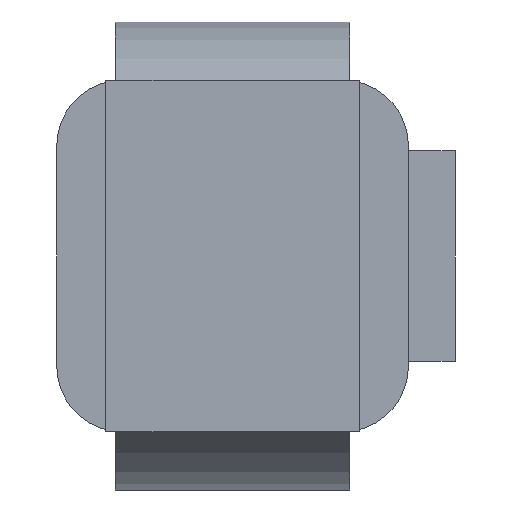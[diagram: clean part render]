
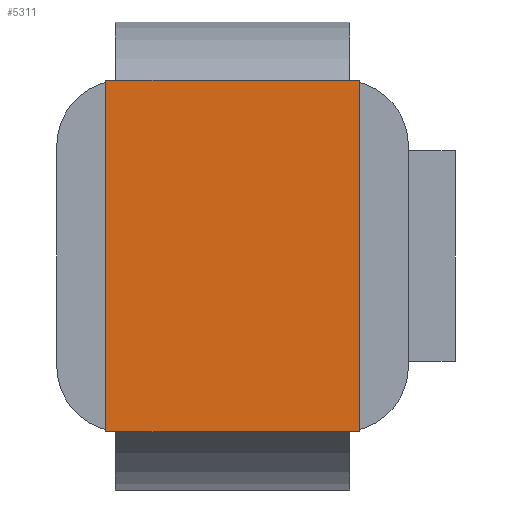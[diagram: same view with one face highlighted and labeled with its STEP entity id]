
A CAD part, front view. The second image highlights one B-rep face of the part: STEP entity #5311.
In plain terms, the highlighted planar face has unit normal (0, -1, 0).
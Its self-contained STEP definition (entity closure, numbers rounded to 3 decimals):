
#1319 = PLANE('',#1320);
#1320 = AXIS2_PLACEMENT_3D('',#1321,#1322,#1323);
#1321 = CARTESIAN_POINT('',(0.,2.6,15.));
#1322 = DIRECTION('',(0.,0.,-1.));
#1323 = DIRECTION('',(-1.,0.,0.));
#1437 = PLANE('',#1438);
#1438 = AXIS2_PLACEMENT_3D('',#1439,#1440,#1441);
#1439 = CARTESIAN_POINT('',(0.,2.6,0.));
#1440 = DIRECTION('',(0.,0.,-1.));
#1441 = DIRECTION('',(-1.,0.,0.));
#2606 = VERTEX_POINT('',#2607);
#2607 = CARTESIAN_POINT('',(3.5,-5.8,0.));
#2621 = PLANE('',#2622);
#2622 = AXIS2_PLACEMENT_3D('',#2623,#2624,#2625);
#2623 = CARTESIAN_POINT('',(3.5,0.,0.));
#2624 = DIRECTION('',(1.,0.,0.));
#2625 = DIRECTION('',(0.,-1.,0.));
#2633 = EDGE_CURVE('',#2606,#2634,#2636,.T.);
#2634 = VERTEX_POINT('',#2635);
#2635 = CARTESIAN_POINT('',(-7.3,-5.8,0.));
#2636 = SURFACE_CURVE('',#2637,(#2641,#2648),.PCURVE_S1.);
#2637 = LINE('',#2638,#2639);
#2638 = CARTESIAN_POINT('',(3.5,-5.8,0.));
#2639 = VECTOR('',#2640,1.);
#2640 = DIRECTION('',(-1.,0.,0.));
#2641 = PCURVE('',#1437,#2642);
#2642 = DEFINITIONAL_REPRESENTATION('',(#2643),#2647);
#2643 = LINE('',#2644,#2645);
#2644 = CARTESIAN_POINT('',(-3.5,-8.4));
#2645 = VECTOR('',#2646,1.);
#2646 = DIRECTION('',(1.,0.));
#2647 = ( GEOMETRIC_REPRESENTATION_CONTEXT(2) 
PARAMETRIC_REPRESENTATION_CONTEXT() REPRESENTATION_CONTEXT('2D SPACE',''
  ) );
#2648 = PCURVE('',#2649,#2654);
#2649 = PLANE('',#2650);
#2650 = AXIS2_PLACEMENT_3D('',#2651,#2652,#2653);
#2651 = CARTESIAN_POINT('',(3.5,-5.8,0.));
#2652 = DIRECTION('',(0.,-1.,0.));
#2653 = DIRECTION('',(-1.,0.,0.));
#2654 = DEFINITIONAL_REPRESENTATION('',(#2655),#2659);
#2655 = LINE('',#2656,#2657);
#2656 = CARTESIAN_POINT('',(0.,0.));
#2657 = VECTOR('',#2658,1.);
#2658 = DIRECTION('',(1.,0.));
#2659 = ( GEOMETRIC_REPRESENTATION_CONTEXT(2) 
PARAMETRIC_REPRESENTATION_CONTEXT() REPRESENTATION_CONTEXT('2D SPACE',''
  ) );
#2677 = PLANE('',#2678);
#2678 = AXIS2_PLACEMENT_3D('',#2679,#2680,#2681);
#2679 = CARTESIAN_POINT('',(-7.3,-5.8,0.));
#2680 = DIRECTION('',(-1.,0.,0.));
#2681 = DIRECTION('',(0.,1.,0.));
#2899 = VERTEX_POINT('',#2900);
#2900 = CARTESIAN_POINT('',(3.5,-5.8,15.));
#2921 = EDGE_CURVE('',#2899,#2922,#2924,.T.);
#2922 = VERTEX_POINT('',#2923);
#2923 = CARTESIAN_POINT('',(-7.3,-5.8,15.));
#2924 = SURFACE_CURVE('',#2925,(#2929,#2936),.PCURVE_S1.);
#2925 = LINE('',#2926,#2927);
#2926 = CARTESIAN_POINT('',(3.5,-5.8,15.));
#2927 = VECTOR('',#2928,1.);
#2928 = DIRECTION('',(-1.,0.,0.));
#2929 = PCURVE('',#1319,#2930);
#2930 = DEFINITIONAL_REPRESENTATION('',(#2931),#2935);
#2931 = LINE('',#2932,#2933);
#2932 = CARTESIAN_POINT('',(-3.5,-8.4));
#2933 = VECTOR('',#2934,1.);
#2934 = DIRECTION('',(1.,0.));
#2935 = ( GEOMETRIC_REPRESENTATION_CONTEXT(2) 
PARAMETRIC_REPRESENTATION_CONTEXT() REPRESENTATION_CONTEXT('2D SPACE',''
  ) );
#2936 = PCURVE('',#2649,#2937);
#2937 = DEFINITIONAL_REPRESENTATION('',(#2938),#2942);
#2938 = LINE('',#2939,#2940);
#2939 = CARTESIAN_POINT('',(0.,-15.));
#2940 = VECTOR('',#2941,1.);
#2941 = DIRECTION('',(1.,0.));
#2942 = ( GEOMETRIC_REPRESENTATION_CONTEXT(2) 
PARAMETRIC_REPRESENTATION_CONTEXT() REPRESENTATION_CONTEXT('2D SPACE',''
  ) );
#5288 = EDGE_CURVE('',#2634,#2922,#5289,.T.);
#5289 = SURFACE_CURVE('',#5290,(#5294,#5301),.PCURVE_S1.);
#5290 = LINE('',#5291,#5292);
#5291 = CARTESIAN_POINT('',(-7.3,-5.8,0.));
#5292 = VECTOR('',#5293,1.);
#5293 = DIRECTION('',(0.,0.,1.));
#5294 = PCURVE('',#2677,#5295);
#5295 = DEFINITIONAL_REPRESENTATION('',(#5296),#5300);
#5296 = LINE('',#5297,#5298);
#5297 = CARTESIAN_POINT('',(0.,0.));
#5298 = VECTOR('',#5299,1.);
#5299 = DIRECTION('',(0.,-1.));
#5300 = ( GEOMETRIC_REPRESENTATION_CONTEXT(2) 
PARAMETRIC_REPRESENTATION_CONTEXT() REPRESENTATION_CONTEXT('2D SPACE',''
  ) );
#5301 = PCURVE('',#2649,#5302);
#5302 = DEFINITIONAL_REPRESENTATION('',(#5303),#5307);
#5303 = LINE('',#5304,#5305);
#5304 = CARTESIAN_POINT('',(10.8,0.));
#5305 = VECTOR('',#5306,1.);
#5306 = DIRECTION('',(0.,-1.));
#5307 = ( GEOMETRIC_REPRESENTATION_CONTEXT(2) 
PARAMETRIC_REPRESENTATION_CONTEXT() REPRESENTATION_CONTEXT('2D SPACE',''
  ) );
#5311 = ADVANCED_FACE('',(#5312),#2649,.T.);
#5312 = FACE_BOUND('',#5313,.T.);
#5313 = EDGE_LOOP('',(#5314,#5335,#5336,#5337));
#5314 = ORIENTED_EDGE('',*,*,#5315,.T.);
#5315 = EDGE_CURVE('',#2606,#2899,#5316,.T.);
#5316 = SURFACE_CURVE('',#5317,(#5321,#5328),.PCURVE_S1.);
#5317 = LINE('',#5318,#5319);
#5318 = CARTESIAN_POINT('',(3.5,-5.8,0.));
#5319 = VECTOR('',#5320,1.);
#5320 = DIRECTION('',(0.,0.,1.));
#5321 = PCURVE('',#2649,#5322);
#5322 = DEFINITIONAL_REPRESENTATION('',(#5323),#5327);
#5323 = LINE('',#5324,#5325);
#5324 = CARTESIAN_POINT('',(0.,0.));
#5325 = VECTOR('',#5326,1.);
#5326 = DIRECTION('',(0.,-1.));
#5327 = ( GEOMETRIC_REPRESENTATION_CONTEXT(2) 
PARAMETRIC_REPRESENTATION_CONTEXT() REPRESENTATION_CONTEXT('2D SPACE',''
  ) );
#5328 = PCURVE('',#2621,#5329);
#5329 = DEFINITIONAL_REPRESENTATION('',(#5330),#5334);
#5330 = LINE('',#5331,#5332);
#5331 = CARTESIAN_POINT('',(5.8,0.));
#5332 = VECTOR('',#5333,1.);
#5333 = DIRECTION('',(0.,-1.));
#5334 = ( GEOMETRIC_REPRESENTATION_CONTEXT(2) 
PARAMETRIC_REPRESENTATION_CONTEXT() REPRESENTATION_CONTEXT('2D SPACE',''
  ) );
#5335 = ORIENTED_EDGE('',*,*,#2921,.T.);
#5336 = ORIENTED_EDGE('',*,*,#5288,.F.);
#5337 = ORIENTED_EDGE('',*,*,#2633,.F.);
